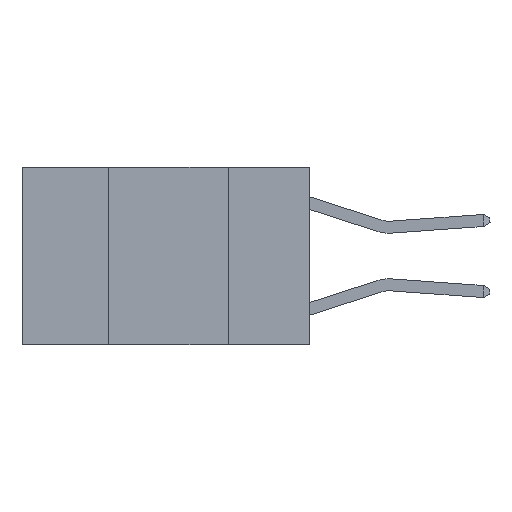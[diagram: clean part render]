
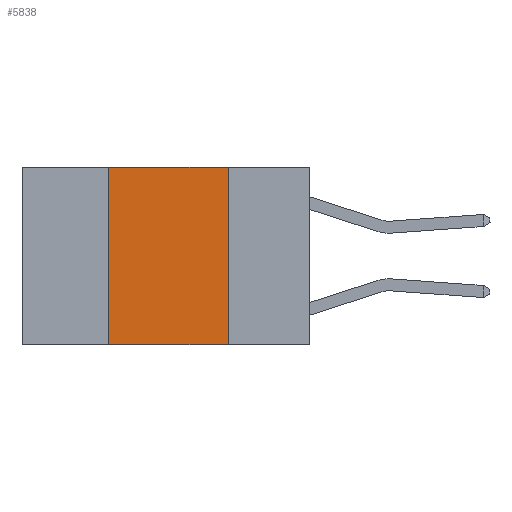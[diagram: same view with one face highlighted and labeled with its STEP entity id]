
A CAD part, left-side view. The second image highlights one B-rep face of the part: STEP entity #5838.
In plain terms, the highlighted planar face has unit normal (-1, 0, 0).
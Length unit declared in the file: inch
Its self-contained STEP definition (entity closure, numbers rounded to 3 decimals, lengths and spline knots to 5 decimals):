
#202 = EDGE_CURVE ( 'NONE', #1371, #10905, #7653, .T. ) ;
#207 = EDGE_CURVE ( 'NONE', #1369, #7516, #9639, .T. ) ;
#219 = EDGE_CURVE ( 'NONE', #1369, #10905, #2795, .T. ) ;
#253 = FACE_OUTER_BOUND ( 'NONE', #8206, .T. ) ;
#1369 = VERTEX_POINT ( 'NONE', #3884 ) ;
#1371 = VERTEX_POINT ( 'NONE', #10847 ) ;
#2210 = AXIS2_PLACEMENT_3D ( 'NONE', #2943, #3861, #10037 ) ;
#2498 = VECTOR ( 'NONE', #7099, 39.37008 ) ;
#2585 = ORIENTED_EDGE ( 'NONE', *, *, #219, .T. ) ;
#2708 = CARTESIAN_POINT ( 'NONE',  ( 0., 0.42, 0. ) ) ;
#2795 = LINE ( 'NONE', #8784, #9374 ) ;
#2943 = CARTESIAN_POINT ( 'NONE',  ( 0., 0.6, 0. ) ) ;
#3085 = VECTOR ( 'NONE', #11187, 39.37008 ) ;
#3861 = DIRECTION ( 'NONE',  ( 1., 0., 0. ) ) ;
#3884 = CARTESIAN_POINT ( 'NONE',  ( 0., 0.42, -0.37 ) ) ;
#4173 = VECTOR ( 'NONE', #7357, 39.37008 ) ;
#4260 = ORIENTED_EDGE ( 'NONE', *, *, #202, .F. ) ;
#4811 = CARTESIAN_POINT ( 'NONE',  ( 0., 0.17, -0.37 ) ) ;
#5251 = CARTESIAN_POINT ( 'NONE',  ( 0., 0.17, 0. ) ) ;
#5838 = ADVANCED_FACE ( 'NONE', ( #253 ), #8361, .F. ) ;
#6545 = ORIENTED_EDGE ( 'NONE', *, *, #207, .F. ) ;
#7099 = DIRECTION ( 'NONE',  ( 0., 0., 1. ) ) ;
#7357 = DIRECTION ( 'NONE',  ( 0., -1., 0. ) ) ;
#7516 = VERTEX_POINT ( 'NONE', #2708 ) ;
#7653 = LINE ( 'NONE', #5251, #3085 ) ;
#7942 = DIRECTION ( 'NONE',  ( 0., -1., 0. ) ) ;
#8206 = EDGE_LOOP ( 'NONE', ( #4260, #10143, #6545, #2585 ) ) ;
#8361 = PLANE ( 'NONE',  #2210 ) ;
#8784 = CARTESIAN_POINT ( 'NONE',  ( 0., 0.6, -0.37 ) ) ;
#9374 = VECTOR ( 'NONE', #7942, 39.37008 ) ;
#9639 = LINE ( 'NONE', #10396, #2498 ) ;
#10037 = DIRECTION ( 'NONE',  ( 0., 0., -1. ) ) ;
#10143 = ORIENTED_EDGE ( 'NONE', *, *, #10694, .F. ) ;
#10396 = CARTESIAN_POINT ( 'NONE',  ( 0., 0.42, 0. ) ) ;
#10694 = EDGE_CURVE ( 'NONE', #7516, #1371, #11095, .T. ) ;
#10847 = CARTESIAN_POINT ( 'NONE',  ( 0., 0.17, 0. ) ) ;
#10905 = VERTEX_POINT ( 'NONE', #4811 ) ;
#11095 = LINE ( 'NONE', #11440, #4173 ) ;
#11187 = DIRECTION ( 'NONE',  ( 0., 0., -1. ) ) ;
#11440 = CARTESIAN_POINT ( 'NONE',  ( 0., 0.6, 0. ) ) ;
